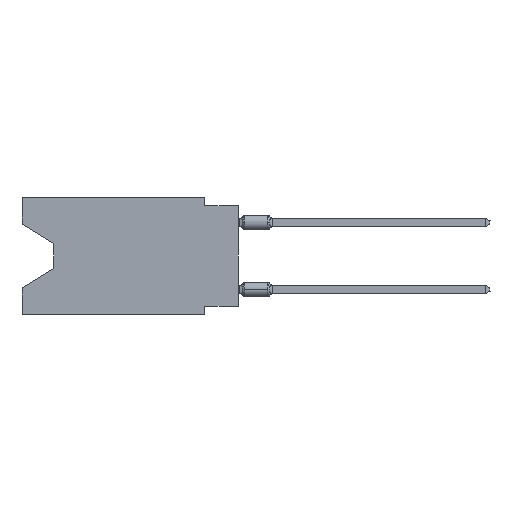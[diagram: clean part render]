
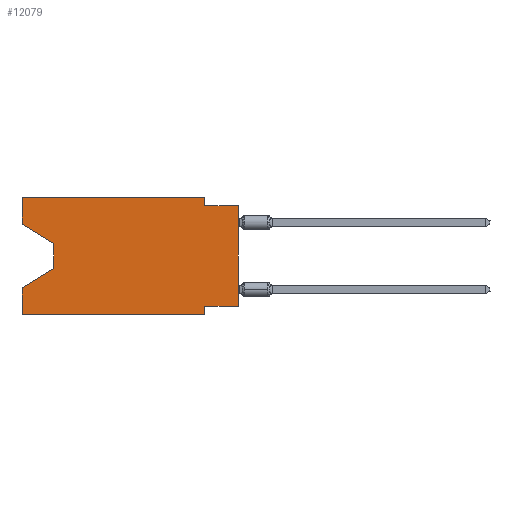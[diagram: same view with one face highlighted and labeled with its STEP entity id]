
A CAD part, left-side view. The second image highlights one B-rep face of the part: STEP entity #12079.
In plain terms, the highlighted planar face has unit normal (-1, 0, 0).
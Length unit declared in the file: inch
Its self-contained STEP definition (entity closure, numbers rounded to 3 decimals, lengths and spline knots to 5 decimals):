
#544 = CARTESIAN_POINT ( 'NONE',  ( 0., 0.645, -0.08025 ) ) ;
#632 = VECTOR ( 'NONE', #17315, 39.37008 ) ;
#1967 = DIRECTION ( 'NONE',  ( 1., 0., 0. ) ) ;
#2322 = PLANE ( 'NONE',  #33036 ) ;
#3108 = VECTOR ( 'NONE', #35190, 39.37008 ) ;
#3576 = ORIENTED_EDGE ( 'NONE', *, *, #24053, .F. ) ;
#3617 = EDGE_CURVE ( 'NONE', #56776, #38262, #6581, .T. ) ;
#3855 = EDGE_CURVE ( 'NONE', #66705, #7093, #14558, .T. ) ;
#3946 = ORIENTED_EDGE ( 'NONE', *, *, #3617, .F. ) ;
#5250 = VECTOR ( 'NONE', #30571, 39.37008 ) ;
#6581 = LINE ( 'NONE', #49185, #62278 ) ;
#7093 = VERTEX_POINT ( 'NONE', #60730 ) ;
#7327 = LINE ( 'NONE', #54858, #23276 ) ;
#7798 = CARTESIAN_POINT ( 'NONE',  ( 0., 0., -0.025 ) ) ;
#8022 = DIRECTION ( 'NONE',  ( 0., 0., -1. ) ) ;
#8622 = CARTESIAN_POINT ( 'NONE',  ( 0., 0.645, -0.08025 ) ) ;
#9140 = VERTEX_POINT ( 'NONE', #37699 ) ;
#9634 = VERTEX_POINT ( 'NONE', #58889 ) ;
#9965 = EDGE_LOOP ( 'NONE', ( #56037, #67267, #66239, #57411, #48707, #59919, #61398, #28256, #3946, #52511, #3576, #19747 ) ) ;
#11492 = VERTEX_POINT ( 'NONE', #39550 ) ;
#11916 = LINE ( 'NONE', #12272, #68827 ) ;
#12079 = ADVANCED_FACE ( 'NONE', ( #50126 ), #2322, .F. ) ;
#12272 = CARTESIAN_POINT ( 'NONE',  ( 0., 0., -0.325 ) ) ;
#13058 = DIRECTION ( 'NONE',  ( 0., 0., -1. ) ) ;
#14558 = LINE ( 'NONE', #8622, #66750 ) ;
#15612 = CARTESIAN_POINT ( 'NONE',  ( 0., 0.645, -0.26975 ) ) ;
#17315 = DIRECTION ( 'NONE',  ( 0., -1., 0. ) ) ;
#17471 = CARTESIAN_POINT ( 'NONE',  ( 0., 0.645, 0. ) ) ;
#17975 = LINE ( 'NONE', #29174, #29919 ) ;
#19669 = CARTESIAN_POINT ( 'NONE',  ( 0., 0.1, -0.025 ) ) ;
#19711 = CARTESIAN_POINT ( 'NONE',  ( 0., 0.645, 0. ) ) ;
#19747 = ORIENTED_EDGE ( 'NONE', *, *, #67903, .F. ) ;
#22406 = LINE ( 'NONE', #17471, #50157 ) ;
#23276 = VECTOR ( 'NONE', #8022, 39.37008 ) ;
#23412 = VECTOR ( 'NONE', #52190, 39.37008 ) ;
#23938 = VERTEX_POINT ( 'NONE', #51870 ) ;
#24053 = EDGE_CURVE ( 'NONE', #65121, #23938, #51525, .T. ) ;
#24716 = LINE ( 'NONE', #66925, #3108 ) ;
#26314 = DIRECTION ( 'NONE',  ( 0., 0., 1. ) ) ;
#28188 = CARTESIAN_POINT ( 'NONE',  ( 0., 0.645, -0.35 ) ) ;
#28256 = ORIENTED_EDGE ( 'NONE', *, *, #66698, .T. ) ;
#29174 = CARTESIAN_POINT ( 'NONE',  ( 0., 0.55, -0.138 ) ) ;
#29919 = VECTOR ( 'NONE', #13058, 39.37008 ) ;
#30571 = DIRECTION ( 'NONE',  ( 0., -1., 0. ) ) ;
#30898 = DIRECTION ( 'NONE',  ( 0., 0., 1. ) ) ;
#31143 = VERTEX_POINT ( 'NONE', #54824 ) ;
#33036 = AXIS2_PLACEMENT_3D ( 'NONE', #39983, #1967, #45558 ) ;
#33306 = CARTESIAN_POINT ( 'NONE',  ( 0., 0.1, -0.325 ) ) ;
#33913 = DIRECTION ( 'NONE',  ( 0., 0., 1. ) ) ;
#35190 = DIRECTION ( 'NONE',  ( 0., 0., -1. ) ) ;
#35432 = LINE ( 'NONE', #52534, #23412 ) ;
#37578 = EDGE_CURVE ( 'NONE', #9140, #42561, #11916, .T. ) ;
#37699 = CARTESIAN_POINT ( 'NONE',  ( 0., 0., -0.325 ) ) ;
#37985 = EDGE_CURVE ( 'NONE', #23938, #56776, #24716, .T. ) ;
#38166 = LINE ( 'NONE', #53562, #45467 ) ;
#38262 = VERTEX_POINT ( 'NONE', #7798 ) ;
#39387 = VERTEX_POINT ( 'NONE', #15612 ) ;
#39550 = CARTESIAN_POINT ( 'NONE',  ( 0., 0.1, -0.35 ) ) ;
#39983 = CARTESIAN_POINT ( 'NONE',  ( 0., 0.645, 0. ) ) ;
#40447 = EDGE_CURVE ( 'NONE', #31143, #39387, #22406, .T. ) ;
#41728 = CARTESIAN_POINT ( 'NONE',  ( 0., 0., 0. ) ) ;
#42561 = VERTEX_POINT ( 'NONE', #33306 ) ;
#43724 = EDGE_CURVE ( 'NONE', #7093, #9634, #17975, .T. ) ;
#43892 = LINE ( 'NONE', #28188, #632 ) ;
#44281 = VECTOR ( 'NONE', #30898, 39.37008 ) ;
#45467 = VECTOR ( 'NONE', #26314, 39.37008 ) ;
#45558 = DIRECTION ( 'NONE',  ( 0., 0., -1. ) ) ;
#46528 = EDGE_CURVE ( 'NONE', #42561, #11492, #7327, .T. ) ;
#47043 = DIRECTION ( 'NONE',  ( 0., -0.855, -0.519 ) ) ;
#48707 = ORIENTED_EDGE ( 'NONE', *, *, #64516, .T. ) ;
#49185 = CARTESIAN_POINT ( 'NONE',  ( 0., 0., -0.025 ) ) ;
#50126 = FACE_OUTER_BOUND ( 'NONE', #9965, .T. ) ;
#50157 = VECTOR ( 'NONE', #33913, 39.37008 ) ;
#51525 = LINE ( 'NONE', #19711, #5250 ) ;
#51603 = EDGE_CURVE ( 'NONE', #9634, #39387, #35432, .T. ) ;
#51870 = CARTESIAN_POINT ( 'NONE',  ( 0., 0.1, 0. ) ) ;
#52190 = DIRECTION ( 'NONE',  ( 0., 0.855, -0.519 ) ) ;
#52511 = ORIENTED_EDGE ( 'NONE', *, *, #37985, .F. ) ;
#52534 = CARTESIAN_POINT ( 'NONE',  ( 0., 0.55, -0.212 ) ) ;
#53562 = CARTESIAN_POINT ( 'NONE',  ( 0., 0.645, 0. ) ) ;
#54212 = DIRECTION ( 'NONE',  ( 0., 1., 0. ) ) ;
#54824 = CARTESIAN_POINT ( 'NONE',  ( 0., 0.645, -0.35 ) ) ;
#54858 = CARTESIAN_POINT ( 'NONE',  ( 0., 0.1, -0.35 ) ) ;
#55312 = CARTESIAN_POINT ( 'NONE',  ( 0., 0.645, 0. ) ) ;
#56037 = ORIENTED_EDGE ( 'NONE', *, *, #3855, .T. ) ;
#56776 = VERTEX_POINT ( 'NONE', #19669 ) ;
#57411 = ORIENTED_EDGE ( 'NONE', *, *, #40447, .F. ) ;
#58889 = CARTESIAN_POINT ( 'NONE',  ( 0., 0.55, -0.212 ) ) ;
#59919 = ORIENTED_EDGE ( 'NONE', *, *, #46528, .F. ) ;
#59954 = DIRECTION ( 'NONE',  ( 0., -1., 0. ) ) ;
#60730 = CARTESIAN_POINT ( 'NONE',  ( 0., 0.55, -0.138 ) ) ;
#61398 = ORIENTED_EDGE ( 'NONE', *, *, #37578, .F. ) ;
#62278 = VECTOR ( 'NONE', #59954, 39.37008 ) ;
#64516 = EDGE_CURVE ( 'NONE', #31143, #11492, #43892, .T. ) ;
#65121 = VERTEX_POINT ( 'NONE', #55312 ) ;
#66239 = ORIENTED_EDGE ( 'NONE', *, *, #51603, .T. ) ;
#66698 = EDGE_CURVE ( 'NONE', #9140, #38262, #68227, .T. ) ;
#66705 = VERTEX_POINT ( 'NONE', #544 ) ;
#66750 = VECTOR ( 'NONE', #47043, 39.37008 ) ;
#66925 = CARTESIAN_POINT ( 'NONE',  ( 0., 0.1, 0. ) ) ;
#67267 = ORIENTED_EDGE ( 'NONE', *, *, #43724, .T. ) ;
#67903 = EDGE_CURVE ( 'NONE', #66705, #65121, #38166, .T. ) ;
#68227 = LINE ( 'NONE', #41728, #44281 ) ;
#68827 = VECTOR ( 'NONE', #54212, 39.37008 ) ;
